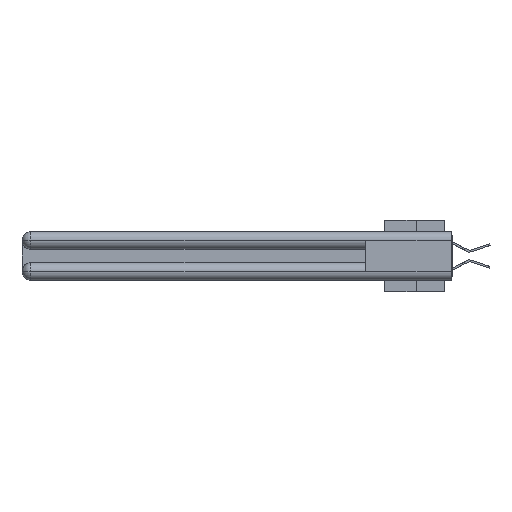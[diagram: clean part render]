
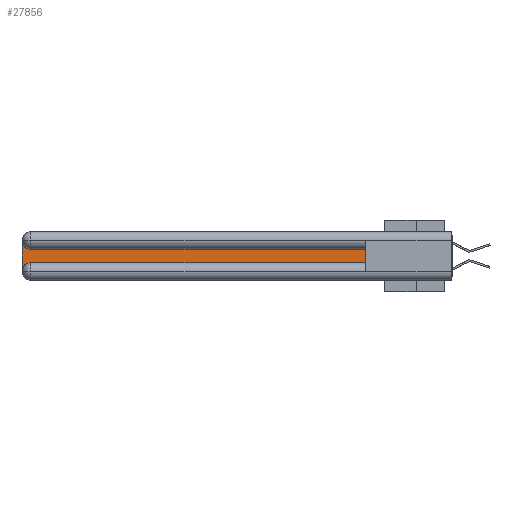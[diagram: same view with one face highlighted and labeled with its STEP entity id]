
A CAD part, left-side view. The second image highlights one B-rep face of the part: STEP entity #27856.
In plain terms, the highlighted planar face has unit normal (-1, 0, 0).
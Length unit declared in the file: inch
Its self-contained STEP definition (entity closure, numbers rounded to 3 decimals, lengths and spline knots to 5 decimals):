
#966 = DIRECTION ( 'NONE',  ( 1., 0., 0. ) ) ;
#1183 = VERTEX_POINT ( 'NONE', #24934 ) ;
#1307 = LINE ( 'NONE', #20111, #26747 ) ;
#2307 = VECTOR ( 'NONE', #18426, 39.37008 ) ;
#2975 = DIRECTION ( 'NONE',  ( 0., 0., -1. ) ) ;
#3146 = DIRECTION ( 'NONE',  ( 1., 0., 0. ) ) ;
#3886 = EDGE_LOOP ( 'NONE', ( #24729, #32556, #17548, #13618, #10880, #24023 ) ) ;
#4250 = VERTEX_POINT ( 'NONE', #9155 ) ;
#5617 = DIRECTION ( 'NONE',  ( 1., 0., 0. ) ) ;
#6124 = CARTESIAN_POINT ( 'NONE',  ( 0.075, 3., -0.2175 ) ) ;
#6232 = CIRCLE ( 'NONE', #23411, 0.06 ) ;
#7736 = DIRECTION ( 'NONE',  ( 0., 0., -1. ) ) ;
#7816 = CARTESIAN_POINT ( 'NONE',  ( 0.075, 0.6, -0.2175 ) ) ;
#8117 = VECTOR ( 'NONE', #8910, 39.37008 ) ;
#8390 = CARTESIAN_POINT ( 'NONE',  ( 0.075, 2.94, -0.2175 ) ) ;
#8628 = VERTEX_POINT ( 'NONE', #27212 ) ;
#8910 = DIRECTION ( 'NONE',  ( 0., 0., -1. ) ) ;
#9140 = DIRECTION ( 'NONE',  ( 0., 1., 0. ) ) ;
#9155 = CARTESIAN_POINT ( 'NONE',  ( 0.075, 3., -0.0625 ) ) ;
#9338 = AXIS2_PLACEMENT_3D ( 'NONE', #28455, #3146, #7736 ) ;
#10880 = ORIENTED_EDGE ( 'NONE', *, *, #20057, .T. ) ;
#11351 = CARTESIAN_POINT ( 'NONE',  ( 0.075, 2.94, -0.0625 ) ) ;
#13000 = VERTEX_POINT ( 'NONE', #32715 ) ;
#13618 = ORIENTED_EDGE ( 'NONE', *, *, #16590, .T. ) ;
#13627 = AXIS2_PLACEMENT_3D ( 'NONE', #27080, #966, #30051 ) ;
#16590 = EDGE_CURVE ( 'NONE', #13000, #18596, #19313, .T. ) ;
#16804 = EDGE_CURVE ( 'NONE', #4250, #13000, #21945, .T. ) ;
#16960 = CARTESIAN_POINT ( 'NONE',  ( 0.075, 0.6, -0.1225 ) ) ;
#17548 = ORIENTED_EDGE ( 'NONE', *, *, #16804, .T. ) ;
#18426 = DIRECTION ( 'NONE',  ( 0., 0., 1. ) ) ;
#18596 = VERTEX_POINT ( 'NONE', #8390 ) ;
#19313 = CIRCLE ( 'NONE', #9338, 0.06 ) ;
#19431 = PLANE ( 'NONE',  #13627 ) ;
#19871 = VERTEX_POINT ( 'NONE', #21678 ) ;
#20057 = EDGE_CURVE ( 'NONE', #18596, #8628, #1307, .T. ) ;
#20111 = CARTESIAN_POINT ( 'NONE',  ( 0.075, 0.6, -0.2175 ) ) ;
#21678 = CARTESIAN_POINT ( 'NONE',  ( 0.075, 0.6, -0.1225 ) ) ;
#21945 = LINE ( 'NONE', #6124, #8117 ) ;
#22029 = EDGE_CURVE ( 'NONE', #1183, #4250, #6232, .T. ) ;
#23411 = AXIS2_PLACEMENT_3D ( 'NONE', #11351, #5617, #2975 ) ;
#23926 = VECTOR ( 'NONE', #9140, 39.37008 ) ;
#24023 = ORIENTED_EDGE ( 'NONE', *, *, #24832, .T. ) ;
#24729 = ORIENTED_EDGE ( 'NONE', *, *, #29743, .T. ) ;
#24787 = LINE ( 'NONE', #16960, #23926 ) ;
#24832 = EDGE_CURVE ( 'NONE', #8628, #19871, #31507, .T. ) ;
#24934 = CARTESIAN_POINT ( 'NONE',  ( 0.075, 2.94, -0.1225 ) ) ;
#26747 = VECTOR ( 'NONE', #30733, 39.37008 ) ;
#27080 = CARTESIAN_POINT ( 'NONE',  ( 0.075, 3., -0.1225 ) ) ;
#27212 = CARTESIAN_POINT ( 'NONE',  ( 0.075, 0.6, -0.2175 ) ) ;
#27613 = FACE_OUTER_BOUND ( 'NONE', #3886, .T. ) ;
#27856 = ADVANCED_FACE ( 'NONE', ( #27613 ), #19431, .F. ) ;
#28455 = CARTESIAN_POINT ( 'NONE',  ( 0.075, 2.94, -0.2775 ) ) ;
#29743 = EDGE_CURVE ( 'NONE', #19871, #1183, #24787, .T. ) ;
#30051 = DIRECTION ( 'NONE',  ( 0., 0., -1. ) ) ;
#30733 = DIRECTION ( 'NONE',  ( 0., -1., 0. ) ) ;
#31507 = LINE ( 'NONE', #7816, #2307 ) ;
#32556 = ORIENTED_EDGE ( 'NONE', *, *, #22029, .T. ) ;
#32715 = CARTESIAN_POINT ( 'NONE',  ( 0.075, 3., -0.2775 ) ) ;
